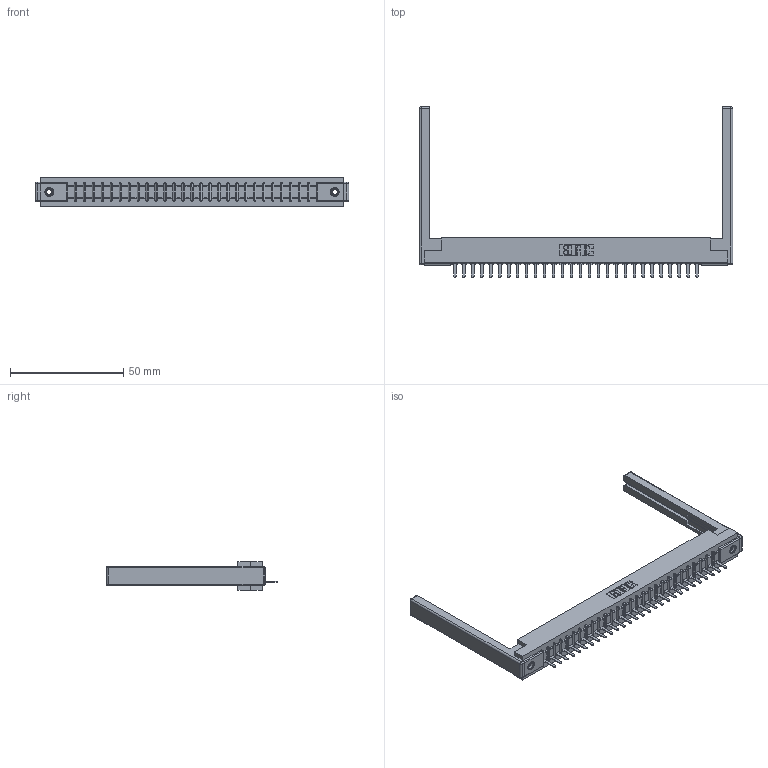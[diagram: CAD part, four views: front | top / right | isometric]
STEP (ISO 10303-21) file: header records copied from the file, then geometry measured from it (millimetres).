
FILE_DESCRIPTION (( 'STEP AP203' ), '1' );
FILE_NAME ('307-028-421-168.STEP', '2020-09-28T07:28:08', ( '' ), ( '' ), 'SwSTEP 2.0', 'SolidWorks 2020', '' );
FILE_SCHEMA (( 'CONFIG_CONTROL_DESIGN' ));
Length unit declared in the file: inch
Products named in the file (5): 307-290-002_521; 307-028-421-168; 307-220-068; 307 Part_.156 Dia Mounting Holes; 345-250-001_345-250-001-102
Assembly tree (33 placements, depth 2):
  307-028-421-168
    307 Part_.156 Dia Mounting Holes
    307-290-002_521  x28
    307-220-068  x2
    345-250-001_345-250-001-102  x2
Bounding box: 138.38 x 75.39 x 12.7 mm (x, y, z)
Volume: 19083.2 mm3; surface area: 22149.5 mm2
Topology: 33 solids, 33 shells, 2373 faces, 7209 edges, 4706 vertices
Faces by surface type: plane 1418, cylinder 873, sphere 66, cone 12, torus 4
Entity records: 29207 total; most frequent: CARTESIAN_POINT 4889, ORIENTED_EDGE 4868, DIRECTION 4774, EDGE_CURVE 2434, LINE 1856, VECTOR 1856, VERTEX_POINT 1574, AXIS2_PLACEMENT_3D 1459
